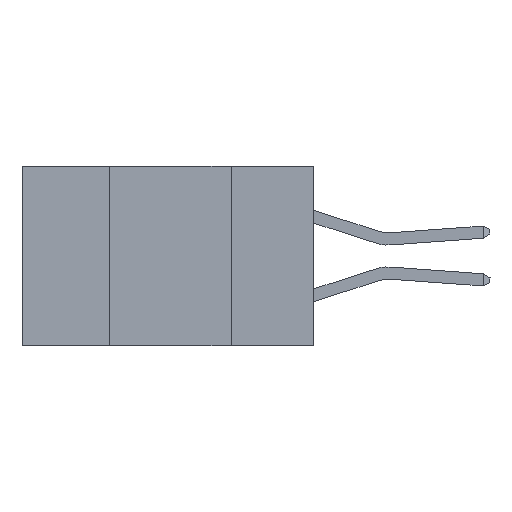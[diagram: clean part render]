
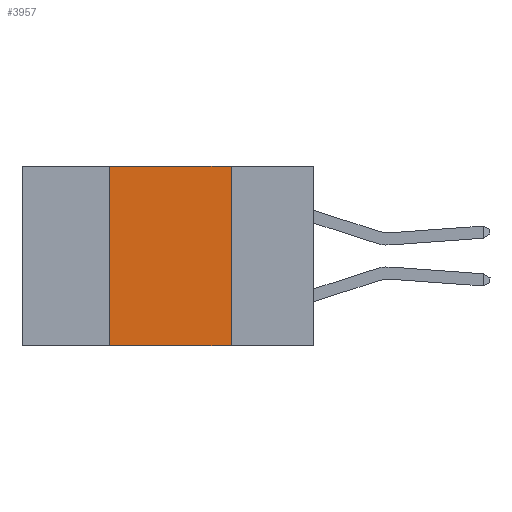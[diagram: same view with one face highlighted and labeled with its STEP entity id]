
A CAD part, left-side view. The second image highlights one B-rep face of the part: STEP entity #3957.
In plain terms, the highlighted planar face has unit normal (-1, 0, 0).
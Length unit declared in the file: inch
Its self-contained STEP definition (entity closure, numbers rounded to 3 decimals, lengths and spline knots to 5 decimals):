
#46 = DIRECTION ( 'NONE',  ( 0., -1., 0. ) ) ;
#170 = FACE_OUTER_BOUND ( 'NONE', #8346, .T. ) ;
#340 = EDGE_CURVE ( 'NONE', #1155, #5026, #3699, .T. ) ;
#504 = CARTESIAN_POINT ( 'NONE',  ( 0., 0.17, -0.37 ) ) ;
#656 = CARTESIAN_POINT ( 'NONE',  ( 0., 0.42, 0. ) ) ;
#729 = CARTESIAN_POINT ( 'NONE',  ( 0., 0.6, 0. ) ) ;
#786 = DIRECTION ( 'NONE',  ( 0., 0., 1. ) ) ;
#1155 = VERTEX_POINT ( 'NONE', #6489 ) ;
#1192 = CARTESIAN_POINT ( 'NONE',  ( 0., 0.42, -0.37 ) ) ;
#1760 = VECTOR ( 'NONE', #9444, 39.37008 ) ;
#1832 = EDGE_CURVE ( 'NONE', #10349, #1155, #9166, .T. ) ;
#2047 = CARTESIAN_POINT ( 'NONE',  ( 0., 0.6, -0.37 ) ) ;
#2976 = LINE ( 'NONE', #2047, #7445 ) ;
#3060 = DIRECTION ( 'NONE',  ( 0., -1., 0. ) ) ;
#3699 = LINE ( 'NONE', #729, #8205 ) ;
#3748 = CARTESIAN_POINT ( 'NONE',  ( 0., 0.17, 0. ) ) ;
#3957 = ADVANCED_FACE ( 'NONE', ( #170 ), #9442, .F. ) ;
#4999 = EDGE_CURVE ( 'NONE', #5026, #7417, #6960, .T. ) ;
#5026 = VERTEX_POINT ( 'NONE', #3748 ) ;
#5692 = EDGE_CURVE ( 'NONE', #10349, #7417, #2976, .T. ) ;
#5870 = ORIENTED_EDGE ( 'NONE', *, *, #340, .F. ) ;
#6489 = CARTESIAN_POINT ( 'NONE',  ( 0., 0.42, 0. ) ) ;
#6960 = LINE ( 'NONE', #7152, #1760 ) ;
#7100 = VECTOR ( 'NONE', #786, 39.37008 ) ;
#7152 = CARTESIAN_POINT ( 'NONE',  ( 0., 0.17, 0. ) ) ;
#7417 = VERTEX_POINT ( 'NONE', #504 ) ;
#7445 = VECTOR ( 'NONE', #3060, 39.37008 ) ;
#8205 = VECTOR ( 'NONE', #46, 39.37008 ) ;
#8346 = EDGE_LOOP ( 'NONE', ( #8714, #5870, #10666, #10111 ) ) ;
#8696 = CARTESIAN_POINT ( 'NONE',  ( 0., 0.6, 0. ) ) ;
#8714 = ORIENTED_EDGE ( 'NONE', *, *, #4999, .F. ) ;
#8801 = AXIS2_PLACEMENT_3D ( 'NONE', #8696, #9875, #10867 ) ;
#9166 = LINE ( 'NONE', #656, #7100 ) ;
#9442 = PLANE ( 'NONE',  #8801 ) ;
#9444 = DIRECTION ( 'NONE',  ( 0., 0., -1. ) ) ;
#9875 = DIRECTION ( 'NONE',  ( 1., 0., 0. ) ) ;
#10111 = ORIENTED_EDGE ( 'NONE', *, *, #5692, .T. ) ;
#10349 = VERTEX_POINT ( 'NONE', #1192 ) ;
#10666 = ORIENTED_EDGE ( 'NONE', *, *, #1832, .F. ) ;
#10867 = DIRECTION ( 'NONE',  ( 0., 0., -1. ) ) ;
